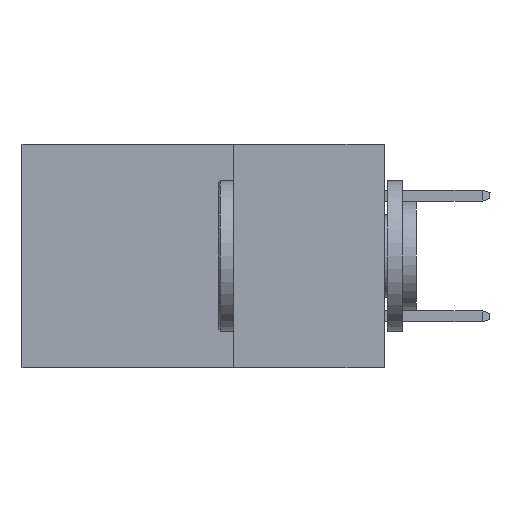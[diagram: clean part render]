
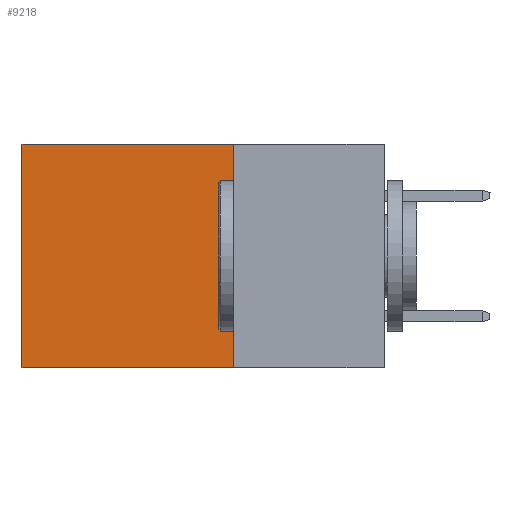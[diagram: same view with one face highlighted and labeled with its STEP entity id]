
A CAD part, left-side view. The second image highlights one B-rep face of the part: STEP entity #9218.
In plain terms, the highlighted planar face has unit normal (-1, 0, 0).
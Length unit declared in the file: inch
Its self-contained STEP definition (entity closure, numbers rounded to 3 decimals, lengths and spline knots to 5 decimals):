
#216 = CARTESIAN_POINT ( 'NONE',  ( 0.298, 0.25, 0. ) ) ;
#1023 = EDGE_CURVE ( 'NONE', #23130, #13125, #9103, .T. ) ;
#1716 = EDGE_CURVE ( 'NONE', #13125, #26485, #28834, .T. ) ;
#3260 = DIRECTION ( 'NONE',  ( 0., 1., 0. ) ) ;
#3487 = CARTESIAN_POINT ( 'NONE',  ( 0.298, 0.25, 0. ) ) ;
#4424 = VECTOR ( 'NONE', #3260, 39.37008 ) ;
#6615 = CARTESIAN_POINT ( 'NONE',  ( 0.298, 0.6, -0.37 ) ) ;
#8618 = CARTESIAN_POINT ( 'NONE',  ( 0.298, 0.6, 0. ) ) ;
#9103 = LINE ( 'NONE', #3487, #4424 ) ;
#9218 = ADVANCED_FACE ( 'NONE', ( #11219 ), #19752, .F. ) ;
#9679 = CARTESIAN_POINT ( 'NONE',  ( 0.298, 0.25, 0. ) ) ;
#9939 = CARTESIAN_POINT ( 'NONE',  ( 0.298, 0.25, -0.37 ) ) ;
#11219 = FACE_OUTER_BOUND ( 'NONE', #14301, .T. ) ;
#11613 = EDGE_CURVE ( 'NONE', #23130, #23144, #23595, .T. ) ;
#13125 = VERTEX_POINT ( 'NONE', #27399 ) ;
#14301 = EDGE_LOOP ( 'NONE', ( #28933, #28714, #16692, #27224 ) ) ;
#14641 = VECTOR ( 'NONE', #21237, 39.37008 ) ;
#14837 = CARTESIAN_POINT ( 'NONE',  ( 0.298, 0.25, 0. ) ) ;
#15985 = DIRECTION ( 'NONE',  ( 0., 1., 0. ) ) ;
#16215 = VECTOR ( 'NONE', #15985, 39.37008 ) ;
#16692 = ORIENTED_EDGE ( 'NONE', *, *, #11613, .F. ) ;
#16827 = DIRECTION ( 'NONE',  ( 0., 0., -1. ) ) ;
#19384 = LINE ( 'NONE', #23421, #16215 ) ;
#19752 = PLANE ( 'NONE',  #27780 ) ;
#20391 = VECTOR ( 'NONE', #16827, 39.37008 ) ;
#21237 = DIRECTION ( 'NONE',  ( 0., 0., -1. ) ) ;
#22148 = EDGE_CURVE ( 'NONE', #23144, #26485, #19384, .T. ) ;
#22953 = DIRECTION ( 'NONE',  ( 1., 0., 0. ) ) ;
#23130 = VERTEX_POINT ( 'NONE', #9679 ) ;
#23144 = VERTEX_POINT ( 'NONE', #9939 ) ;
#23421 = CARTESIAN_POINT ( 'NONE',  ( 0.298, 0.25, -0.37 ) ) ;
#23595 = LINE ( 'NONE', #14837, #20391 ) ;
#26485 = VERTEX_POINT ( 'NONE', #6615 ) ;
#27224 = ORIENTED_EDGE ( 'NONE', *, *, #1023, .T. ) ;
#27399 = CARTESIAN_POINT ( 'NONE',  ( 0.298, 0.6, 0. ) ) ;
#27780 = AXIS2_PLACEMENT_3D ( 'NONE', #216, #22953, #32539 ) ;
#28714 = ORIENTED_EDGE ( 'NONE', *, *, #22148, .F. ) ;
#28834 = LINE ( 'NONE', #8618, #14641 ) ;
#28933 = ORIENTED_EDGE ( 'NONE', *, *, #1716, .T. ) ;
#32539 = DIRECTION ( 'NONE',  ( 0., 0., -1. ) ) ;
